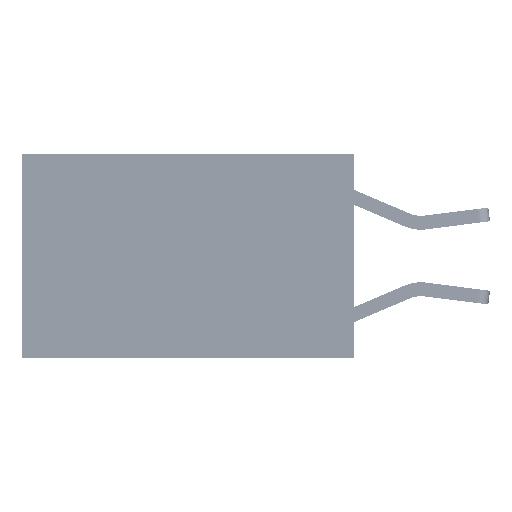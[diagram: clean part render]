
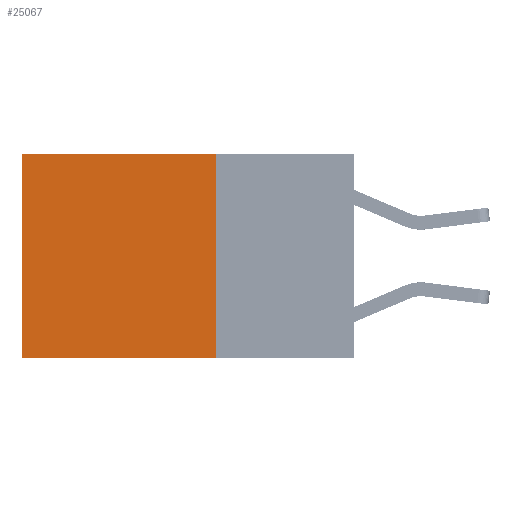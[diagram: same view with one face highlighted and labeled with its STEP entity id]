
A CAD part, left-side view. The second image highlights one B-rep face of the part: STEP entity #25067.
In plain terms, the highlighted planar face has unit normal (-1, 0, 0).
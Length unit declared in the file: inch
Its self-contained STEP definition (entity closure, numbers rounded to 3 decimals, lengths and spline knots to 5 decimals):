
#28 = VERTEX_POINT ( 'NONE', #13302 ) ;
#925 = CARTESIAN_POINT ( 'NONE',  ( 0.2625, 0.6, 0. ) ) ;
#1420 = DIRECTION ( 'NONE',  ( 0., 1., 0. ) ) ;
#1557 = EDGE_CURVE ( 'NONE', #2775, #23614, #17682, .T. ) ;
#2775 = VERTEX_POINT ( 'NONE', #19640 ) ;
#3211 = LINE ( 'NONE', #20625, #10504 ) ;
#3795 = PLANE ( 'NONE',  #27881 ) ;
#3815 = LINE ( 'NONE', #13639, #22213 ) ;
#6407 = VERTEX_POINT ( 'NONE', #26730 ) ;
#10504 = VECTOR ( 'NONE', #1420, 39.37008 ) ;
#10892 = DIRECTION ( 'NONE',  ( 0., 0., -1. ) ) ;
#10981 = CARTESIAN_POINT ( 'NONE',  ( 0.2625, 0.6, -0.37 ) ) ;
#12350 = EDGE_CURVE ( 'NONE', #6407, #28, #27423, .T. ) ;
#12526 = ORIENTED_EDGE ( 'NONE', *, *, #12350, .F. ) ;
#12585 = CARTESIAN_POINT ( 'NONE',  ( 0.2625, 0.25, 0. ) ) ;
#13302 = CARTESIAN_POINT ( 'NONE',  ( 0.2625, 0.25, -0.37 ) ) ;
#13617 = DIRECTION ( 'NONE',  ( 1., 0., 0. ) ) ;
#13639 = CARTESIAN_POINT ( 'NONE',  ( 0.2625, 0.25, -0.37 ) ) ;
#17682 = LINE ( 'NONE', #925, #27549 ) ;
#19640 = CARTESIAN_POINT ( 'NONE',  ( 0.2625, 0.6, 0. ) ) ;
#20625 = CARTESIAN_POINT ( 'NONE',  ( 0.2625, 0.25, 0. ) ) ;
#21356 = DIRECTION ( 'NONE',  ( 0., 0., -1. ) ) ;
#22213 = VECTOR ( 'NONE', #23472, 39.37008 ) ;
#22283 = DIRECTION ( 'NONE',  ( 0., 0., -1. ) ) ;
#23368 = EDGE_CURVE ( 'NONE', #28, #23614, #3815, .T. ) ;
#23472 = DIRECTION ( 'NONE',  ( 0., 1., 0. ) ) ;
#23614 = VERTEX_POINT ( 'NONE', #10981 ) ;
#24207 = ORIENTED_EDGE ( 'NONE', *, *, #1557, .T. ) ;
#24470 = EDGE_LOOP ( 'NONE', ( #24207, #25969, #12526, #30883 ) ) ;
#25067 = ADVANCED_FACE ( 'NONE', ( #28295 ), #3795, .F. ) ;
#25969 = ORIENTED_EDGE ( 'NONE', *, *, #23368, .F. ) ;
#26059 = VECTOR ( 'NONE', #22283, 39.37008 ) ;
#26340 = CARTESIAN_POINT ( 'NONE',  ( 0.2625, 0.25, 0. ) ) ;
#26730 = CARTESIAN_POINT ( 'NONE',  ( 0.2625, 0.25, 0. ) ) ;
#27423 = LINE ( 'NONE', #12585, #26059 ) ;
#27549 = VECTOR ( 'NONE', #10892, 39.37008 ) ;
#27881 = AXIS2_PLACEMENT_3D ( 'NONE', #26340, #13617, #21356 ) ;
#28295 = FACE_OUTER_BOUND ( 'NONE', #24470, .T. ) ;
#29040 = EDGE_CURVE ( 'NONE', #6407, #2775, #3211, .T. ) ;
#30883 = ORIENTED_EDGE ( 'NONE', *, *, #29040, .T. ) ;
